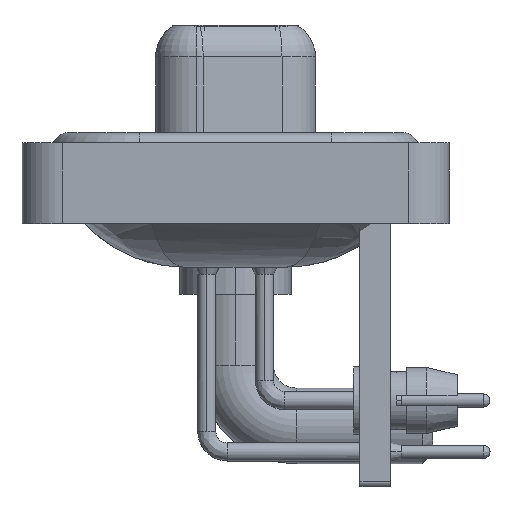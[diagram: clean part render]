
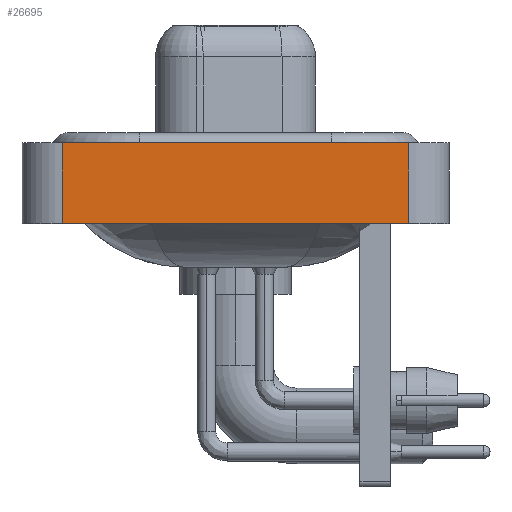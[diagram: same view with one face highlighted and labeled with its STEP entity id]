
A CAD part, left-side view. The second image highlights one B-rep face of the part: STEP entity #26695.
In plain terms, the highlighted planar face has unit normal (-1, 0, 0).
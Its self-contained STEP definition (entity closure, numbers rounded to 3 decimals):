
#330 = VERTEX_POINT ( 'NONE', #9211 ) ;
#898 = VERTEX_POINT ( 'NONE', #14165 ) ;
#1105 = DIRECTION ( 'NONE',  ( 0., -1., 0. ) ) ;
#1809 = VERTEX_POINT ( 'NONE', #6031 ) ;
#2296 = EDGE_CURVE ( 'NONE', #25387, #898, #19679, .T. ) ;
#2703 = VECTOR ( 'NONE', #4369, 1000. ) ;
#3016 = LINE ( 'NONE', #11764, #12663 ) ;
#4369 = DIRECTION ( 'NONE',  ( 0., -1., 0. ) ) ;
#4631 = PLANE ( 'NONE',  #28570 ) ;
#5179 = CARTESIAN_POINT ( 'NONE',  ( -7.35, 8.55, -3.6 ) ) ;
#5397 = EDGE_CURVE ( 'NONE', #330, #1809, #3016, .T. ) ;
#5867 = LINE ( 'NONE', #16526, #6570 ) ;
#6031 = CARTESIAN_POINT ( 'NONE',  ( -7.35, -8.55, 0.4 ) ) ;
#6139 = ORIENTED_EDGE ( 'NONE', *, *, #2296, .T. ) ;
#6570 = VECTOR ( 'NONE', #9649, 1000. ) ;
#9211 = CARTESIAN_POINT ( 'NONE',  ( -7.35, 8.55, 0.4 ) ) ;
#9492 = LINE ( 'NONE', #18410, #25260 ) ;
#9649 = DIRECTION ( 'NONE',  ( 0., 0., 1. ) ) ;
#10919 = CARTESIAN_POINT ( 'NONE',  ( -7.35, -8.55, -3.6 ) ) ;
#11764 = CARTESIAN_POINT ( 'NONE',  ( -7.35, -8.55, 0.4 ) ) ;
#12663 = VECTOR ( 'NONE', #1105, 1000. ) ;
#13525 = DIRECTION ( 'NONE',  ( -1., 0., 0. ) ) ;
#14165 = CARTESIAN_POINT ( 'NONE',  ( -7.35, -8.55, -3.6 ) ) ;
#14931 = EDGE_CURVE ( 'NONE', #898, #1809, #5867, .T. ) ;
#15841 = FACE_OUTER_BOUND ( 'NONE', #22196, .T. ) ;
#16526 = CARTESIAN_POINT ( 'NONE',  ( -7.35, -8.55, -3.6 ) ) ;
#17070 = EDGE_CURVE ( 'NONE', #25387, #330, #9492, .T. ) ;
#17757 = DIRECTION ( 'NONE',  ( 0., 0., 1. ) ) ;
#18410 = CARTESIAN_POINT ( 'NONE',  ( -7.35, 8.55, -3.6 ) ) ;
#19679 = LINE ( 'NONE', #10919, #2703 ) ;
#22196 = EDGE_LOOP ( 'NONE', ( #26307, #25634, #25315, #6139 ) ) ;
#22648 = DIRECTION ( 'NONE',  ( 0., 0., 1. ) ) ;
#25260 = VECTOR ( 'NONE', #22648, 1000. ) ;
#25315 = ORIENTED_EDGE ( 'NONE', *, *, #17070, .F. ) ;
#25387 = VERTEX_POINT ( 'NONE', #5179 ) ;
#25634 = ORIENTED_EDGE ( 'NONE', *, *, #5397, .F. ) ;
#26307 = ORIENTED_EDGE ( 'NONE', *, *, #14931, .T. ) ;
#26639 = CARTESIAN_POINT ( 'NONE',  ( -7.35, -8.55, -3.6 ) ) ;
#26695 = ADVANCED_FACE ( 'NONE', ( #15841 ), #4631, .T. ) ;
#28570 = AXIS2_PLACEMENT_3D ( 'NONE', #26639, #13525, #17757 ) ;
